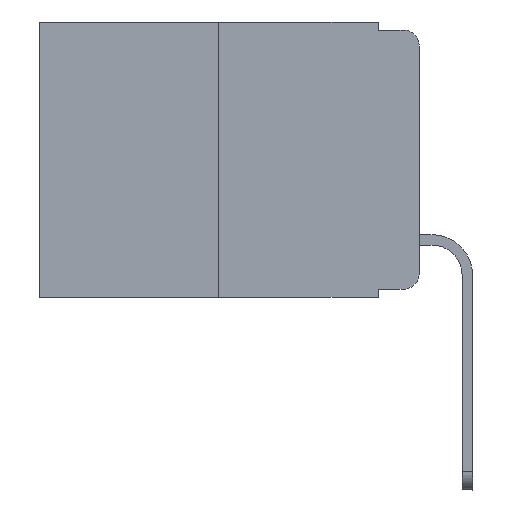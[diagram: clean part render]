
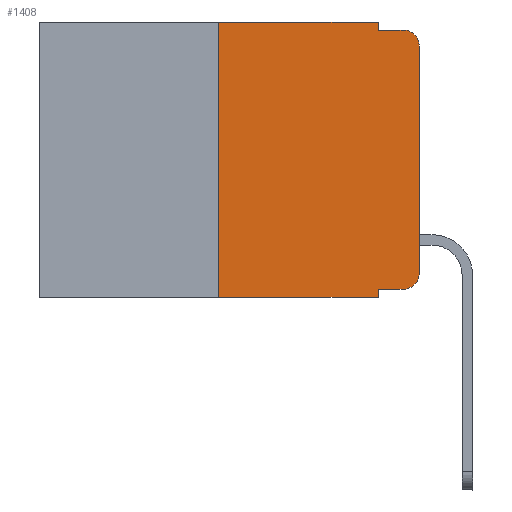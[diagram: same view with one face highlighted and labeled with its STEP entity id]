
A CAD part, left-side view. The second image highlights one B-rep face of the part: STEP entity #1408.
In plain terms, the highlighted planar face has unit normal (-1, 0, 0).
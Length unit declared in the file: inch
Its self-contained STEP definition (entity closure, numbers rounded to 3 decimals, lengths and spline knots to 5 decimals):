
#24 = AXIS2_PLACEMENT_3D ( 'NONE', #8724, #6099, #11365 ) ;
#156 = VERTEX_POINT ( 'NONE', #975 ) ;
#224 = VECTOR ( 'NONE', #7787, 39.37008 ) ;
#450 = DIRECTION ( 'NONE',  ( 0., 0., 1. ) ) ;
#463 = VERTEX_POINT ( 'NONE', #5250 ) ;
#501 = CARTESIAN_POINT ( 'NONE',  ( 0., 0.051, 0. ) ) ;
#579 = DIRECTION ( 'NONE',  ( 0., 0., -1. ) ) ;
#603 = EDGE_CURVE ( 'NONE', #8037, #463, #4294, .T. ) ;
#635 = CARTESIAN_POINT ( 'NONE',  ( 0., 0.051, 0. ) ) ;
#648 = DIRECTION ( 'NONE',  ( 0., -1., 0. ) ) ;
#843 = EDGE_CURVE ( 'NONE', #993, #156, #1318, .T. ) ;
#854 = EDGE_CURVE ( 'NONE', #10313, #1501, #3109, .T. ) ;
#894 = ORIENTED_EDGE ( 'NONE', *, *, #843, .F. ) ;
#963 = ORIENTED_EDGE ( 'NONE', *, *, #1442, .F. ) ;
#975 = CARTESIAN_POINT ( 'NONE',  ( 0., 0.051, -0.01 ) ) ;
#993 = VERTEX_POINT ( 'NONE', #501 ) ;
#1033 = VECTOR ( 'NONE', #450, 39.37008 ) ;
#1068 = ORIENTED_EDGE ( 'NONE', *, *, #7964, .T. ) ;
#1318 = LINE ( 'NONE', #4837, #2345 ) ;
#1408 = ADVANCED_FACE ( 'NONE', ( #3319 ), #2488, .F. ) ;
#1442 = EDGE_CURVE ( 'NONE', #1501, #993, #8668, .T. ) ;
#1463 = CARTESIAN_POINT ( 'NONE',  ( 0., 0.473, -0.343 ) ) ;
#1501 = VERTEX_POINT ( 'NONE', #8784 ) ;
#1840 = CARTESIAN_POINT ( 'NONE',  ( 0., 0., 0. ) ) ;
#2345 = VECTOR ( 'NONE', #8456, 39.37008 ) ;
#2488 = PLANE ( 'NONE',  #24 ) ;
#2706 = VERTEX_POINT ( 'NONE', #10232 ) ;
#2784 = CARTESIAN_POINT ( 'NONE',  ( 0., 0., -0.03 ) ) ;
#2858 = DIRECTION ( 'NONE',  ( 0., 0., 1. ) ) ;
#3066 = DIRECTION ( 'NONE',  ( 0., 0., -1. ) ) ;
#3109 = LINE ( 'NONE', #4947, #1033 ) ;
#3150 = ORIENTED_EDGE ( 'NONE', *, *, #5712, .F. ) ;
#3184 = ORIENTED_EDGE ( 'NONE', *, *, #6726, .T. ) ;
#3319 = FACE_OUTER_BOUND ( 'NONE', #11198, .T. ) ;
#3409 = CARTESIAN_POINT ( 'NONE',  ( 0., 0.051, -0.333 ) ) ;
#3937 = ORIENTED_EDGE ( 'NONE', *, *, #8822, .T. ) ;
#4052 = EDGE_CURVE ( 'NONE', #10313, #6984, #4488, .T. ) ;
#4294 = LINE ( 'NONE', #3409, #8374 ) ;
#4488 = LINE ( 'NONE', #1463, #224 ) ;
#4748 = AXIS2_PLACEMENT_3D ( 'NONE', #8251, #5509, #7314 ) ;
#4817 = CARTESIAN_POINT ( 'NONE',  ( 0., 0.051, -0.343 ) ) ;
#4837 = CARTESIAN_POINT ( 'NONE',  ( 0., 0.051, 0. ) ) ;
#4947 = CARTESIAN_POINT ( 'NONE',  ( 0., 0.25, 0. ) ) ;
#5019 = CARTESIAN_POINT ( 'NONE',  ( 0., 0.02, -0.313 ) ) ;
#5250 = CARTESIAN_POINT ( 'NONE',  ( 0., 0.02, -0.333 ) ) ;
#5509 = DIRECTION ( 'NONE',  ( -1., 0., 0. ) ) ;
#5690 = VECTOR ( 'NONE', #648, 39.37008 ) ;
#5712 = EDGE_CURVE ( 'NONE', #8037, #6984, #8712, .T. ) ;
#5845 = DIRECTION ( 'NONE',  ( 0., -1., 0. ) ) ;
#5960 = DIRECTION ( 'NONE',  ( 0., -1., 0. ) ) ;
#6059 = CIRCLE ( 'NONE', #4748, 0.02 ) ;
#6099 = DIRECTION ( 'NONE',  ( 1., 0., 0. ) ) ;
#6239 = VECTOR ( 'NONE', #2858, 39.37008 ) ;
#6291 = ORIENTED_EDGE ( 'NONE', *, *, #854, .F. ) ;
#6647 = CARTESIAN_POINT ( 'NONE',  ( 0., 0.25, -0.343 ) ) ;
#6710 = EDGE_CURVE ( 'NONE', #156, #2706, #7540, .T. ) ;
#6726 = EDGE_CURVE ( 'NONE', #463, #8051, #10316, .T. ) ;
#6949 = AXIS2_PLACEMENT_3D ( 'NONE', #5019, #11228, #3066 ) ;
#6984 = VERTEX_POINT ( 'NONE', #4817 ) ;
#7136 = ORIENTED_EDGE ( 'NONE', *, *, #6710, .F. ) ;
#7314 = DIRECTION ( 'NONE',  ( 0., 0., -1. ) ) ;
#7540 = LINE ( 'NONE', #10224, #11625 ) ;
#7787 = DIRECTION ( 'NONE',  ( 0., -1., 0. ) ) ;
#7816 = CARTESIAN_POINT ( 'NONE',  ( 0., 0.051, -0.333 ) ) ;
#7964 = EDGE_CURVE ( 'NONE', #10605, #2706, #6059, .T. ) ;
#8037 = VERTEX_POINT ( 'NONE', #7816 ) ;
#8051 = VERTEX_POINT ( 'NONE', #11286 ) ;
#8251 = CARTESIAN_POINT ( 'NONE',  ( 0., 0.02, -0.03 ) ) ;
#8374 = VECTOR ( 'NONE', #5960, 39.37008 ) ;
#8456 = DIRECTION ( 'NONE',  ( 0., 0., -1. ) ) ;
#8568 = VECTOR ( 'NONE', #579, 39.37008 ) ;
#8580 = ORIENTED_EDGE ( 'NONE', *, *, #603, .T. ) ;
#8668 = LINE ( 'NONE', #10368, #5690 ) ;
#8712 = LINE ( 'NONE', #635, #8568 ) ;
#8724 = CARTESIAN_POINT ( 'NONE',  ( 0., 0.473, 0. ) ) ;
#8784 = CARTESIAN_POINT ( 'NONE',  ( 0., 0.25, 0. ) ) ;
#8822 = EDGE_CURVE ( 'NONE', #8051, #10605, #10792, .T. ) ;
#10224 = CARTESIAN_POINT ( 'NONE',  ( 0., 0.051, -0.01 ) ) ;
#10232 = CARTESIAN_POINT ( 'NONE',  ( 0., 0.02, -0.01 ) ) ;
#10313 = VERTEX_POINT ( 'NONE', #6647 ) ;
#10316 = CIRCLE ( 'NONE', #6949, 0.02 ) ;
#10368 = CARTESIAN_POINT ( 'NONE',  ( 0., 0.473, 0. ) ) ;
#10605 = VERTEX_POINT ( 'NONE', #2784 ) ;
#10792 = LINE ( 'NONE', #1840, #6239 ) ;
#11198 = EDGE_LOOP ( 'NONE', ( #3937, #1068, #7136, #894, #963, #6291, #11296, #3150, #8580, #3184 ) ) ;
#11228 = DIRECTION ( 'NONE',  ( -1., 0., 0. ) ) ;
#11286 = CARTESIAN_POINT ( 'NONE',  ( 0., 0., -0.313 ) ) ;
#11296 = ORIENTED_EDGE ( 'NONE', *, *, #4052, .T. ) ;
#11365 = DIRECTION ( 'NONE',  ( 0., 0., -1. ) ) ;
#11625 = VECTOR ( 'NONE', #5845, 39.37008 ) ;
